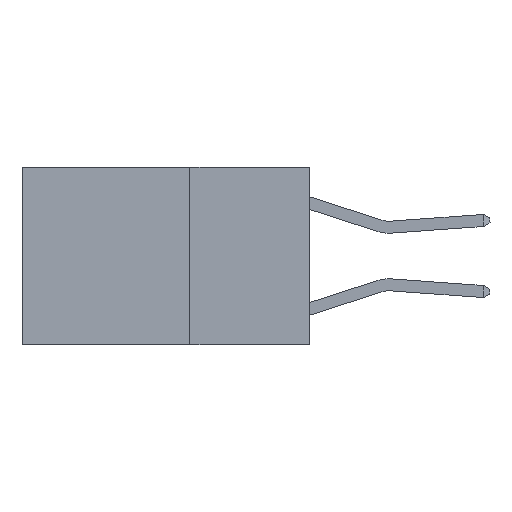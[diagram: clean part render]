
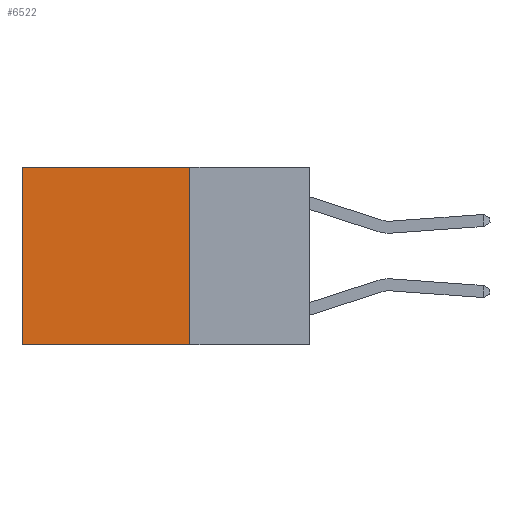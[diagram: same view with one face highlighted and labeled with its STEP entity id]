
A CAD part, left-side view. The second image highlights one B-rep face of the part: STEP entity #6522.
In plain terms, the highlighted planar face has unit normal (-1, 0, 0).
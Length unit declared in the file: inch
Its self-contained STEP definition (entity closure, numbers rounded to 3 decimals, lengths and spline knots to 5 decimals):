
#176 = LINE ( 'NONE', #9192, #8443 ) ;
#337 = DIRECTION ( 'NONE',  ( 0., 0., -1. ) ) ;
#1722 = VERTEX_POINT ( 'NONE', #2609 ) ;
#1793 = VERTEX_POINT ( 'NONE', #8774 ) ;
#2298 = CARTESIAN_POINT ( 'NONE',  ( 0.2625, 0.25, 0. ) ) ;
#2609 = CARTESIAN_POINT ( 'NONE',  ( 0.2625, 0.25, -0.37 ) ) ;
#2650 = ORIENTED_EDGE ( 'NONE', *, *, #6507, .T. ) ;
#3123 = CARTESIAN_POINT ( 'NONE',  ( 0.2625, 0.6, 0. ) ) ;
#3914 = DIRECTION ( 'NONE',  ( 0., 1., 0. ) ) ;
#4214 = VECTOR ( 'NONE', #7258, 39.37008 ) ;
#4307 = CARTESIAN_POINT ( 'NONE',  ( 0.2625, 0.25, 0. ) ) ;
#4512 = FACE_OUTER_BOUND ( 'NONE', #10267, .T. ) ;
#4862 = AXIS2_PLACEMENT_3D ( 'NONE', #2298, #7021, #11999 ) ;
#4967 = VECTOR ( 'NONE', #3914, 39.37008 ) ;
#5617 = ORIENTED_EDGE ( 'NONE', *, *, #10696, .T. ) ;
#5949 = VERTEX_POINT ( 'NONE', #12478 ) ;
#6507 = EDGE_CURVE ( 'NONE', #1793, #7363, #11828, .T. ) ;
#6522 = ADVANCED_FACE ( 'NONE', ( #4512 ), #10134, .F. ) ;
#7021 = DIRECTION ( 'NONE',  ( 1., 0., 0. ) ) ;
#7068 = ORIENTED_EDGE ( 'NONE', *, *, #7971, .F. ) ;
#7102 = DIRECTION ( 'NONE',  ( 0., 0., -1. ) ) ;
#7258 = DIRECTION ( 'NONE',  ( 0., 1., 0. ) ) ;
#7363 = VERTEX_POINT ( 'NONE', #11111 ) ;
#7585 = LINE ( 'NONE', #7794, #4967 ) ;
#7794 = CARTESIAN_POINT ( 'NONE',  ( 0.2625, 0.25, -0.37 ) ) ;
#7971 = EDGE_CURVE ( 'NONE', #5949, #1722, #176, .T. ) ;
#8443 = VECTOR ( 'NONE', #337, 39.37008 ) ;
#8774 = CARTESIAN_POINT ( 'NONE',  ( 0.2625, 0.6, 0. ) ) ;
#9192 = CARTESIAN_POINT ( 'NONE',  ( 0.2625, 0.25, 0. ) ) ;
#9426 = LINE ( 'NONE', #4307, #4214 ) ;
#10134 = PLANE ( 'NONE',  #4862 ) ;
#10267 = EDGE_LOOP ( 'NONE', ( #2650, #11816, #7068, #5617 ) ) ;
#10696 = EDGE_CURVE ( 'NONE', #5949, #1793, #9426, .T. ) ;
#11111 = CARTESIAN_POINT ( 'NONE',  ( 0.2625, 0.6, -0.37 ) ) ;
#11713 = EDGE_CURVE ( 'NONE', #1722, #7363, #7585, .T. ) ;
#11816 = ORIENTED_EDGE ( 'NONE', *, *, #11713, .F. ) ;
#11828 = LINE ( 'NONE', #3123, #11975 ) ;
#11975 = VECTOR ( 'NONE', #7102, 39.37008 ) ;
#11999 = DIRECTION ( 'NONE',  ( 0., 0., -1. ) ) ;
#12478 = CARTESIAN_POINT ( 'NONE',  ( 0.2625, 0.25, 0. ) ) ;
